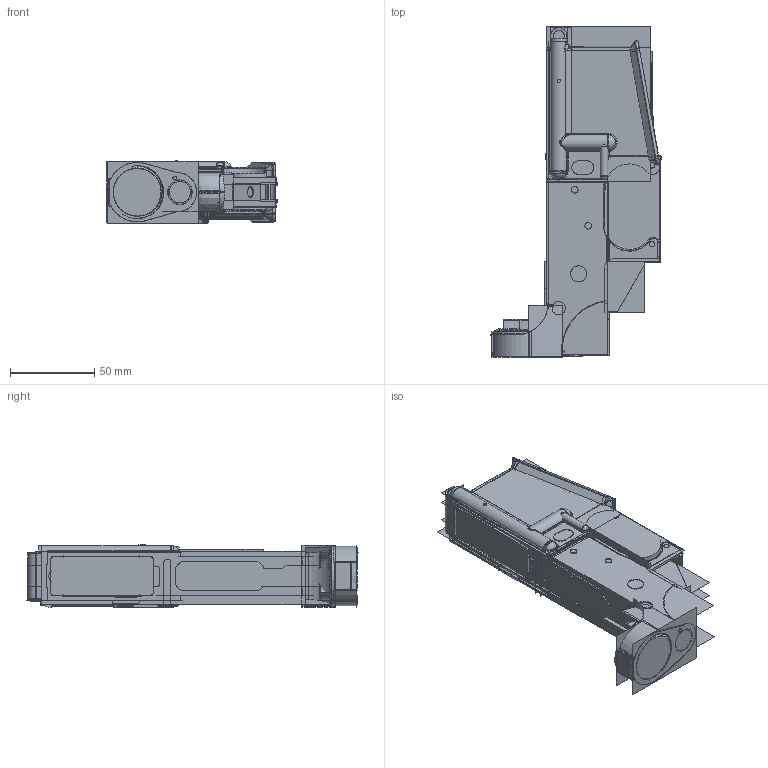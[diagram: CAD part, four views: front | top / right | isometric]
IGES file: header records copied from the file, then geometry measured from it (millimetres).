
Start section:  PTC IGES file: ar15lwrmach_asm.igs
Global section: file name: ar15lwrmach_asm.igs; native system: Pro/ENGINEER by Parametric Technology Corporation; preprocessor: 9906; author: EMD2492; organization: Unknown; date: 000225.070109; units: inch
Bounding box: 101.03 x 197.26 x 37.93 mm (x, y, z)
Surface area: 248108.1 mm2 (no closed solid volume)
Topology: 0 solids, 0 shells, 982 faces, 12018 edges, 13902 vertices
Faces by surface type: revolution 548, bspline 434
